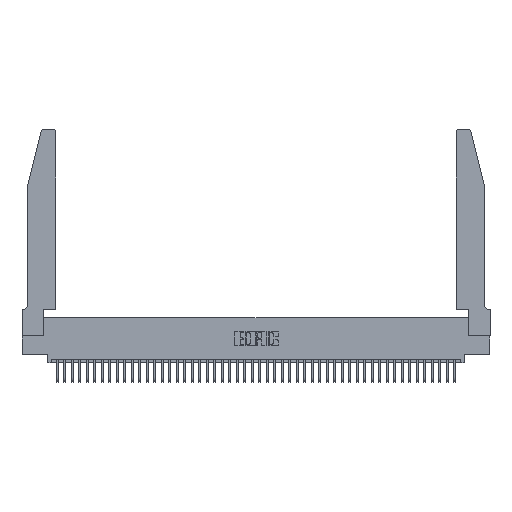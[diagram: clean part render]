
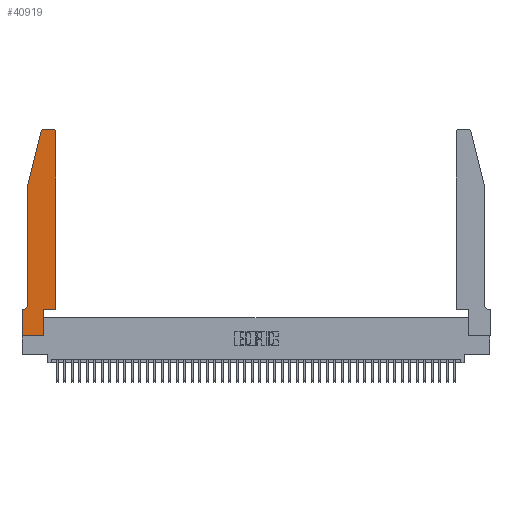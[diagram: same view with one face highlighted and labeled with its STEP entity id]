
A CAD part, top view. The second image highlights one B-rep face of the part: STEP entity #40919.
In plain terms, the highlighted planar face has unit normal (0, 0, 1).
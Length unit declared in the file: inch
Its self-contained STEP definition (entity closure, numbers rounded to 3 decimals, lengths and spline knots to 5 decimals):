
#131 = CARTESIAN_POINT ( 'NONE',  ( 0.4205, 2.75, 0.37 ) ) ;
#482 = ORIENTED_EDGE ( 'NONE', *, *, #25056, .T. ) ;
#946 = ORIENTED_EDGE ( 'NONE', *, *, #20166, .T. ) ;
#974 = LINE ( 'NONE', #23575, #3785 ) ;
#1820 = DIRECTION ( 'NONE',  ( 0., 0., 1. ) ) ;
#1895 = CARTESIAN_POINT ( 'NONE',  ( 0., 0.35, 0.37 ) ) ;
#3649 = CARTESIAN_POINT ( 'NONE',  ( 0.0755, 0.35, 0.37 ) ) ;
#3785 = VECTOR ( 'NONE', #16693, 39.37008 ) ;
#3993 = DIRECTION ( 'NONE',  ( 0., 0., 1. ) ) ;
#4124 = EDGE_CURVE ( 'NONE', #19455, #5189, #6636, .T. ) ;
#4597 = CARTESIAN_POINT ( 'NONE',  ( 0.4505, 2.72, 0.37 ) ) ;
#4749 = DIRECTION ( 'NONE',  ( 0., 1., 0. ) ) ;
#5050 = VERTEX_POINT ( 'NONE', #8295 ) ;
#5189 = VERTEX_POINT ( 'NONE', #34866 ) ;
#5400 = ORIENTED_EDGE ( 'NONE', *, *, #44737, .T. ) ;
#5452 = EDGE_LOOP ( 'NONE', ( #14102, #32702, #20591, #29342, #43868, #18411, #5400, #26705, #482, #43918, #8039, #946 ) ) ;
#5588 = PLANE ( 'NONE',  #34893 ) ;
#6098 = DIRECTION ( 'NONE',  ( 1., 0., 0. ) ) ;
#6636 = LINE ( 'NONE', #3649, #15820 ) ;
#7870 = CARTESIAN_POINT ( 'NONE',  ( 0.0755, 2., 0.37 ) ) ;
#8039 = ORIENTED_EDGE ( 'NONE', *, *, #28603, .T. ) ;
#8295 = CARTESIAN_POINT ( 'NONE',  ( 0.0755, 2., 0.37 ) ) ;
#8419 = EDGE_CURVE ( 'NONE', #31965, #12926, #32686, .T. ) ;
#8646 = CARTESIAN_POINT ( 'NONE',  ( 0.2865, 0., 0.37 ) ) ;
#8795 = DIRECTION ( 'NONE',  ( 1., 0., 0. ) ) ;
#8885 = CARTESIAN_POINT ( 'NONE',  ( 0.4505, 0.35, 0.37 ) ) ;
#9679 = AXIS2_PLACEMENT_3D ( 'NONE', #34742, #1820, #27850 ) ;
#10597 = EDGE_CURVE ( 'NONE', #10886, #19455, #11276, .T. ) ;
#10886 = VERTEX_POINT ( 'NONE', #16560 ) ;
#11003 = DIRECTION ( 'NONE',  ( -1., 0., 0. ) ) ;
#11276 = CIRCLE ( 'NONE', #43980, 0.07 ) ;
#11436 = VERTEX_POINT ( 'NONE', #40014 ) ;
#11525 = CARTESIAN_POINT ( 'NONE',  ( 0.4505, 0.35, 0.37 ) ) ;
#12192 = LINE ( 'NONE', #17686, #33951 ) ;
#12926 = VERTEX_POINT ( 'NONE', #47121 ) ;
#13232 = VECTOR ( 'NONE', #24741, 39.37008 ) ;
#13677 = DIRECTION ( 'NONE',  ( 0., -1., 0. ) ) ;
#13832 = CARTESIAN_POINT ( 'NONE',  ( 0.0755, 2., 0.37 ) ) ;
#14024 = CARTESIAN_POINT ( 'NONE',  ( 0.4505, 0.35, 0.37 ) ) ;
#14102 = ORIENTED_EDGE ( 'NONE', *, *, #8419, .T. ) ;
#15820 = VECTOR ( 'NONE', #11003, 39.37008 ) ;
#16560 = CARTESIAN_POINT ( 'NONE',  ( 0.0755, 0.42, 0.37 ) ) ;
#16587 = CARTESIAN_POINT ( 'NONE',  ( 0.0055, 0.35, 0.37 ) ) ;
#16662 = CARTESIAN_POINT ( 'NONE',  ( 0.0055, 0.42, 0.37 ) ) ;
#16693 = DIRECTION ( 'NONE',  ( 0., 1., 0. ) ) ;
#17003 = LINE ( 'NONE', #8885, #24957 ) ;
#17235 = VECTOR ( 'NONE', #8795, 39.37008 ) ;
#17682 = VERTEX_POINT ( 'NONE', #21178 ) ;
#17686 = CARTESIAN_POINT ( 'NONE',  ( 0., 0., 0.37 ) ) ;
#18193 = CARTESIAN_POINT ( 'NONE',  ( 0.2865, 0.35, 0.37 ) ) ;
#18411 = ORIENTED_EDGE ( 'NONE', *, *, #4124, .T. ) ;
#18417 = DIRECTION ( 'NONE',  ( -0.239, -0.971, 0. ) ) ;
#19455 = VERTEX_POINT ( 'NONE', #16587 ) ;
#20166 = EDGE_CURVE ( 'NONE', #20463, #31965, #29954, .T. ) ;
#20463 = VERTEX_POINT ( 'NONE', #4597 ) ;
#20591 = ORIENTED_EDGE ( 'NONE', *, *, #43601, .T. ) ;
#21178 = CARTESIAN_POINT ( 'NONE',  ( 0., 0., 0.37 ) ) ;
#21359 = EDGE_CURVE ( 'NONE', #12926, #11436, #45292, .T. ) ;
#22247 = LINE ( 'NONE', #14024, #34284 ) ;
#23575 = CARTESIAN_POINT ( 'NONE',  ( 0.2865, 0.35, 0.37 ) ) ;
#24741 = DIRECTION ( 'NONE',  ( -1., 0., 0. ) ) ;
#24957 = VECTOR ( 'NONE', #4749, 39.37008 ) ;
#25010 = DIRECTION ( 'NONE',  ( 0., -1., 0. ) ) ;
#25056 = EDGE_CURVE ( 'NONE', #40156, #33614, #974, .T. ) ;
#25386 = VERTEX_POINT ( 'NONE', #11525 ) ;
#26705 = ORIENTED_EDGE ( 'NONE', *, *, #40311, .T. ) ;
#26954 = LINE ( 'NONE', #34853, #17235 ) ;
#27372 = DIRECTION ( 'NONE',  ( 0., 0., -1. ) ) ;
#27451 = DIRECTION ( 'NONE',  ( 0., 0., 1. ) ) ;
#27850 = DIRECTION ( 'NONE',  ( 1., 0., 0. ) ) ;
#28330 = VECTOR ( 'NONE', #18417, 39.37008 ) ;
#28603 = EDGE_CURVE ( 'NONE', #25386, #20463, #17003, .T. ) ;
#29342 = ORIENTED_EDGE ( 'NONE', *, *, #42754, .T. ) ;
#29954 = CIRCLE ( 'NONE', #34502, 0.03 ) ;
#31871 = VECTOR ( 'NONE', #13677, 39.37008 ) ;
#31965 = VERTEX_POINT ( 'NONE', #131 ) ;
#32316 = LINE ( 'NONE', #7870, #28330 ) ;
#32686 = LINE ( 'NONE', #35464, #13232 ) ;
#32702 = ORIENTED_EDGE ( 'NONE', *, *, #21359, .T. ) ;
#33562 = EDGE_CURVE ( 'NONE', #33614, #25386, #22247, .T. ) ;
#33614 = VERTEX_POINT ( 'NONE', #18193 ) ;
#33751 = FACE_OUTER_BOUND ( 'NONE', #5452, .T. ) ;
#33951 = VECTOR ( 'NONE', #25010, 39.37008 ) ;
#34284 = VECTOR ( 'NONE', #6098, 39.37008 ) ;
#34502 = AXIS2_PLACEMENT_3D ( 'NONE', #40751, #3993, #40268 ) ;
#34742 = CARTESIAN_POINT ( 'NONE',  ( 0.284, 2.72, 0.37 ) ) ;
#34853 = CARTESIAN_POINT ( 'NONE',  ( 0., 0., 0.37 ) ) ;
#34866 = CARTESIAN_POINT ( 'NONE',  ( 0., 0.35, 0.37 ) ) ;
#34893 = AXIS2_PLACEMENT_3D ( 'NONE', #1895, #27451, #45666 ) ;
#35464 = CARTESIAN_POINT ( 'NONE',  ( 0.2605, 2.75, 0.37 ) ) ;
#40014 = CARTESIAN_POINT ( 'NONE',  ( 0.25487, 2.72718, 0.37 ) ) ;
#40156 = VERTEX_POINT ( 'NONE', #8646 ) ;
#40268 = DIRECTION ( 'NONE',  ( 1., 0., 0. ) ) ;
#40311 = EDGE_CURVE ( 'NONE', #17682, #40156, #26954, .T. ) ;
#40751 = CARTESIAN_POINT ( 'NONE',  ( 0.4205, 2.72, 0.37 ) ) ;
#40919 = ADVANCED_FACE ( 'NONE', ( #33751 ), #5588, .T. ) ;
#42211 = DIRECTION ( 'NONE',  ( -1., 0., 0. ) ) ;
#42754 = EDGE_CURVE ( 'NONE', #5050, #10886, #45579, .T. ) ;
#43601 = EDGE_CURVE ( 'NONE', #11436, #5050, #32316, .T. ) ;
#43868 = ORIENTED_EDGE ( 'NONE', *, *, #10597, .T. ) ;
#43918 = ORIENTED_EDGE ( 'NONE', *, *, #33562, .T. ) ;
#43980 = AXIS2_PLACEMENT_3D ( 'NONE', #16662, #27372, #42211 ) ;
#44737 = EDGE_CURVE ( 'NONE', #5189, #17682, #12192, .T. ) ;
#45292 = CIRCLE ( 'NONE', #9679, 0.03 ) ;
#45579 = LINE ( 'NONE', #13832, #31871 ) ;
#45666 = DIRECTION ( 'NONE',  ( 1., 0., 0. ) ) ;
#47121 = CARTESIAN_POINT ( 'NONE',  ( 0.284, 2.75, 0.37 ) ) ;
